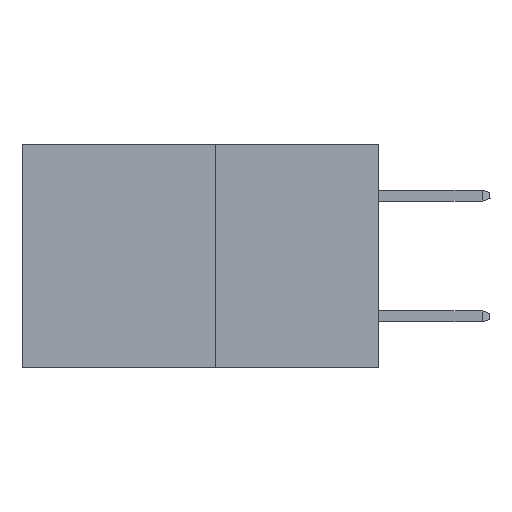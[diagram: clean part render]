
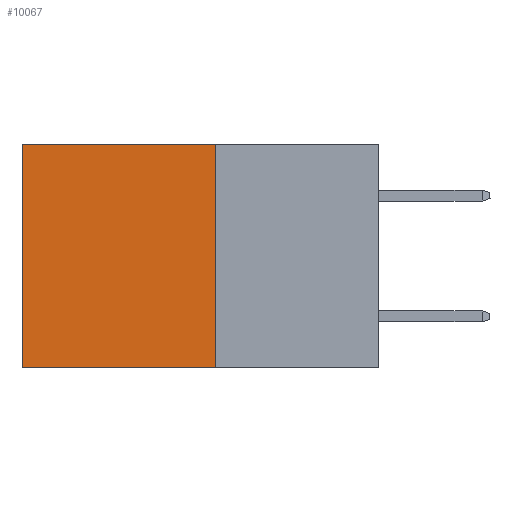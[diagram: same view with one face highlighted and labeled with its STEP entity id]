
A CAD part, left-side view. The second image highlights one B-rep face of the part: STEP entity #10067.
In plain terms, the highlighted planar face has unit normal (-1, 0, 0).
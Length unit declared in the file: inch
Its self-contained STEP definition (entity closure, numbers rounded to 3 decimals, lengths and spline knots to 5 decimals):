
#1574 = CARTESIAN_POINT ( 'NONE',  ( 0.277, 0.27, -0.37 ) ) ;
#2232 = CARTESIAN_POINT ( 'NONE',  ( 0.277, 0.27, 0. ) ) ;
#2373 = VECTOR ( 'NONE', #3872, 39.37008 ) ;
#3107 = ORIENTED_EDGE ( 'NONE', *, *, #14616, .T. ) ;
#3277 = ORIENTED_EDGE ( 'NONE', *, *, #6892, .F. ) ;
#3403 = ORIENTED_EDGE ( 'NONE', *, *, #5704, .F. ) ;
#3450 = DIRECTION ( 'NONE',  ( 0., 1., 0. ) ) ;
#3561 = ORIENTED_EDGE ( 'NONE', *, *, #5081, .T. ) ;
#3872 = DIRECTION ( 'NONE',  ( 0., 1., 0. ) ) ;
#4746 = VERTEX_POINT ( 'NONE', #12996 ) ;
#4818 = VERTEX_POINT ( 'NONE', #15384 ) ;
#5081 = EDGE_CURVE ( 'NONE', #17790, #4818, #19218, .T. ) ;
#5704 = EDGE_CURVE ( 'NONE', #17790, #4746, #17712, .T. ) ;
#6620 = VECTOR ( 'NONE', #3450, 39.37008 ) ;
#6892 = EDGE_CURVE ( 'NONE', #4746, #15746, #11027, .T. ) ;
#8910 = DIRECTION ( 'NONE',  ( 0., 0., -1. ) ) ;
#9707 = CARTESIAN_POINT ( 'NONE',  ( 0.277, 0.27, -0.37 ) ) ;
#10067 = ADVANCED_FACE ( 'NONE', ( #16649 ), #15664, .F. ) ;
#11027 = LINE ( 'NONE', #15578, #2373 ) ;
#12996 = CARTESIAN_POINT ( 'NONE',  ( 0.277, 0.27, -0.37 ) ) ;
#13004 = VECTOR ( 'NONE', #8910, 39.37008 ) ;
#13751 = AXIS2_PLACEMENT_3D ( 'NONE', #1574, #15635, #15631 ) ;
#14616 = EDGE_CURVE ( 'NONE', #4818, #15746, #17218, .T. ) ;
#15384 = CARTESIAN_POINT ( 'NONE',  ( 0.277, 0.59, 0. ) ) ;
#15578 = CARTESIAN_POINT ( 'NONE',  ( 0.277, 0.27, -0.37 ) ) ;
#15631 = DIRECTION ( 'NONE',  ( 0., 0., -1. ) ) ;
#15635 = DIRECTION ( 'NONE',  ( 1., 0., 0. ) ) ;
#15664 = PLANE ( 'NONE',  #13751 ) ;
#15746 = VERTEX_POINT ( 'NONE', #16589 ) ;
#16589 = CARTESIAN_POINT ( 'NONE',  ( 0.277, 0.59, -0.37 ) ) ;
#16649 = FACE_OUTER_BOUND ( 'NONE', #16984, .T. ) ;
#16984 = EDGE_LOOP ( 'NONE', ( #3107, #3277, #3403, #3561 ) ) ;
#17218 = LINE ( 'NONE', #18921, #17721 ) ;
#17712 = LINE ( 'NONE', #9707, #13004 ) ;
#17721 = VECTOR ( 'NONE', #18903, 39.37008 ) ;
#17790 = VERTEX_POINT ( 'NONE', #20808 ) ;
#18903 = DIRECTION ( 'NONE',  ( 0., 0., -1. ) ) ;
#18921 = CARTESIAN_POINT ( 'NONE',  ( 0.277, 0.59, -0.37 ) ) ;
#19218 = LINE ( 'NONE', #2232, #6620 ) ;
#20808 = CARTESIAN_POINT ( 'NONE',  ( 0.277, 0.27, 0. ) ) ;
